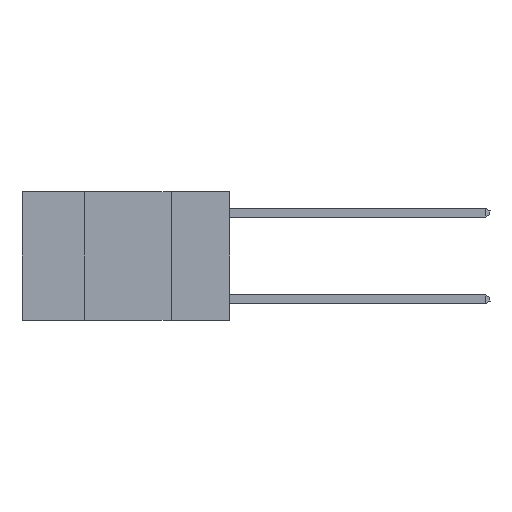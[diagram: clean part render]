
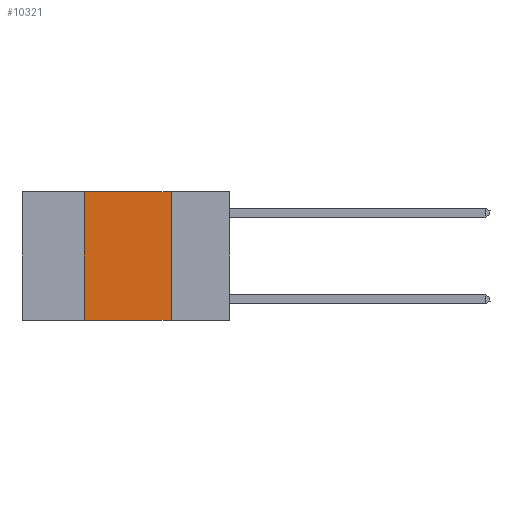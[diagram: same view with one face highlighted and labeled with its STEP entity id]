
A CAD part, left-side view. The second image highlights one B-rep face of the part: STEP entity #10321.
In plain terms, the highlighted planar face has unit normal (-1, 0, 0).
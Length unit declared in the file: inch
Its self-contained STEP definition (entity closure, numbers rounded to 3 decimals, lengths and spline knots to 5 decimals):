
#75 = PLANE ( 'NONE',  #11565 ) ;
#489 = CARTESIAN_POINT ( 'NONE',  ( 0., 0.6, 0. ) ) ;
#932 = VERTEX_POINT ( 'NONE', #9609 ) ;
#996 = ORIENTED_EDGE ( 'NONE', *, *, #6899, .T. ) ;
#1262 = CARTESIAN_POINT ( 'NONE',  ( 0., 0.42, 0. ) ) ;
#2316 = EDGE_CURVE ( 'NONE', #8201, #4047, #9326, .T. ) ;
#2493 = ORIENTED_EDGE ( 'NONE', *, *, #5006, .F. ) ;
#2518 = LINE ( 'NONE', #489, #4379 ) ;
#3500 = CARTESIAN_POINT ( 'NONE',  ( 0., 0.42, -0.37 ) ) ;
#3763 = CARTESIAN_POINT ( 'NONE',  ( 0., 0.6, -0.37 ) ) ;
#4004 = VECTOR ( 'NONE', #11448, 39.37008 ) ;
#4047 = VERTEX_POINT ( 'NONE', #11112 ) ;
#4312 = VECTOR ( 'NONE', #5159, 39.37008 ) ;
#4379 = VECTOR ( 'NONE', #10178, 39.37008 ) ;
#5006 = EDGE_CURVE ( 'NONE', #4047, #10207, #2518, .T. ) ;
#5159 = DIRECTION ( 'NONE',  ( 0., 0., 1. ) ) ;
#5591 = LINE ( 'NONE', #3763, #6925 ) ;
#6632 = EDGE_LOOP ( 'NONE', ( #10729, #2493, #10025, #996 ) ) ;
#6899 = EDGE_CURVE ( 'NONE', #8201, #932, #5591, .T. ) ;
#6925 = VECTOR ( 'NONE', #10355, 39.37008 ) ;
#7852 = DIRECTION ( 'NONE',  ( 1., 0., 0. ) ) ;
#8201 = VERTEX_POINT ( 'NONE', #3500 ) ;
#8336 = EDGE_CURVE ( 'NONE', #10207, #932, #11308, .T. ) ;
#8525 = CARTESIAN_POINT ( 'NONE',  ( 0., 0.17, 0. ) ) ;
#8607 = CARTESIAN_POINT ( 'NONE',  ( 0., 0.6, 0. ) ) ;
#9326 = LINE ( 'NONE', #1262, #4312 ) ;
#9609 = CARTESIAN_POINT ( 'NONE',  ( 0., 0.17, -0.37 ) ) ;
#10025 = ORIENTED_EDGE ( 'NONE', *, *, #2316, .F. ) ;
#10178 = DIRECTION ( 'NONE',  ( 0., -1., 0. ) ) ;
#10207 = VERTEX_POINT ( 'NONE', #11978 ) ;
#10321 = ADVANCED_FACE ( 'NONE', ( #11591 ), #75, .F. ) ;
#10355 = DIRECTION ( 'NONE',  ( 0., -1., 0. ) ) ;
#10729 = ORIENTED_EDGE ( 'NONE', *, *, #8336, .F. ) ;
#11112 = CARTESIAN_POINT ( 'NONE',  ( 0., 0.42, 0. ) ) ;
#11308 = LINE ( 'NONE', #8525, #4004 ) ;
#11448 = DIRECTION ( 'NONE',  ( 0., 0., -1. ) ) ;
#11565 = AXIS2_PLACEMENT_3D ( 'NONE', #8607, #7852, #11704 ) ;
#11591 = FACE_OUTER_BOUND ( 'NONE', #6632, .T. ) ;
#11704 = DIRECTION ( 'NONE',  ( 0., 0., -1. ) ) ;
#11978 = CARTESIAN_POINT ( 'NONE',  ( 0., 0.17, 0. ) ) ;
